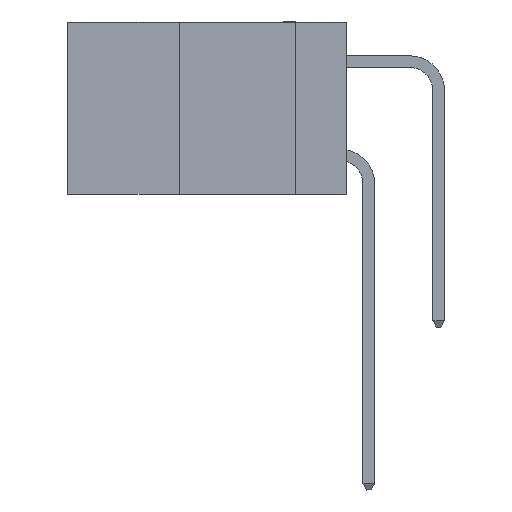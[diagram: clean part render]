
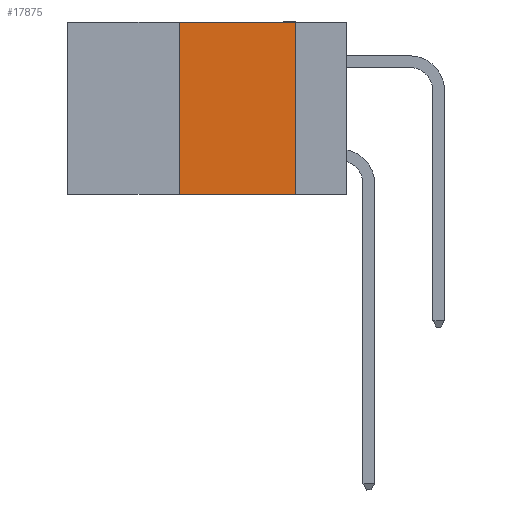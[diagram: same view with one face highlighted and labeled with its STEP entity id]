
A CAD part, left-side view. The second image highlights one B-rep face of the part: STEP entity #17875.
In plain terms, the highlighted planar face has unit normal (-1, 0, 0).
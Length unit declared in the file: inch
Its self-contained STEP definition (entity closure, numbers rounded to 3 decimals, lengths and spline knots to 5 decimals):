
#288 = DIRECTION ( 'NONE',  ( 0., -1., 0. ) ) ;
#866 = PLANE ( 'NONE',  #20729 ) ;
#1017 = CARTESIAN_POINT ( 'NONE',  ( 0., 0.6, 0. ) ) ;
#1438 = ORIENTED_EDGE ( 'NONE', *, *, #19950, .T. ) ;
#3087 = LINE ( 'NONE', #25857, #4327 ) ;
#4327 = VECTOR ( 'NONE', #288, 39.37008 ) ;
#4459 = VERTEX_POINT ( 'NONE', #29430 ) ;
#5775 = ORIENTED_EDGE ( 'NONE', *, *, #12130, .F. ) ;
#6870 = VECTOR ( 'NONE', #14717, 39.37008 ) ;
#8740 = DIRECTION ( 'NONE',  ( 0., 0., -1. ) ) ;
#11068 = EDGE_CURVE ( 'NONE', #4459, #15825, #20272, .T. ) ;
#12130 = EDGE_CURVE ( 'NONE', #26978, #14871, #13699, .T. ) ;
#12817 = FACE_OUTER_BOUND ( 'NONE', #32184, .T. ) ;
#13699 = LINE ( 'NONE', #29013, #22370 ) ;
#14544 = ORIENTED_EDGE ( 'NONE', *, *, #11068, .F. ) ;
#14717 = DIRECTION ( 'NONE',  ( 0., -1., 0. ) ) ;
#14871 = VERTEX_POINT ( 'NONE', #24477 ) ;
#15417 = EDGE_CURVE ( 'NONE', #15825, #26978, #24761, .T. ) ;
#15825 = VERTEX_POINT ( 'NONE', #27490 ) ;
#15915 = DIRECTION ( 'NONE',  ( 0., 0., -1. ) ) ;
#16075 = DIRECTION ( 'NONE',  ( 1., 0., 0. ) ) ;
#17875 = ADVANCED_FACE ( 'NONE', ( #12817 ), #866, .F. ) ;
#19507 = ORIENTED_EDGE ( 'NONE', *, *, #15417, .F. ) ;
#19692 = CARTESIAN_POINT ( 'NONE',  ( 0., 0.6, 0. ) ) ;
#19950 = EDGE_CURVE ( 'NONE', #4459, #14871, #3087, .T. ) ;
#20272 = LINE ( 'NONE', #30283, #25551 ) ;
#20729 = AXIS2_PLACEMENT_3D ( 'NONE', #1017, #16075, #15915 ) ;
#22370 = VECTOR ( 'NONE', #8740, 39.37008 ) ;
#22872 = DIRECTION ( 'NONE',  ( 0., 0., 1. ) ) ;
#24477 = CARTESIAN_POINT ( 'NONE',  ( 0., 0.11, -0.37 ) ) ;
#24761 = LINE ( 'NONE', #19692, #6870 ) ;
#25551 = VECTOR ( 'NONE', #22872, 39.37008 ) ;
#25857 = CARTESIAN_POINT ( 'NONE',  ( 0., 0.6, -0.37 ) ) ;
#26978 = VERTEX_POINT ( 'NONE', #27897 ) ;
#27490 = CARTESIAN_POINT ( 'NONE',  ( 0., 0.36, 0. ) ) ;
#27897 = CARTESIAN_POINT ( 'NONE',  ( 0., 0.11, 0. ) ) ;
#29013 = CARTESIAN_POINT ( 'NONE',  ( 0., 0.11, 0. ) ) ;
#29430 = CARTESIAN_POINT ( 'NONE',  ( 0., 0.36, -0.37 ) ) ;
#30283 = CARTESIAN_POINT ( 'NONE',  ( 0., 0.36, 0. ) ) ;
#32184 = EDGE_LOOP ( 'NONE', ( #5775, #19507, #14544, #1438 ) ) ;
